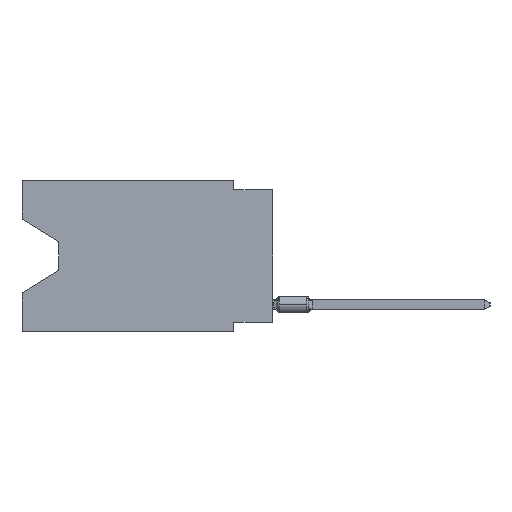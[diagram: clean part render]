
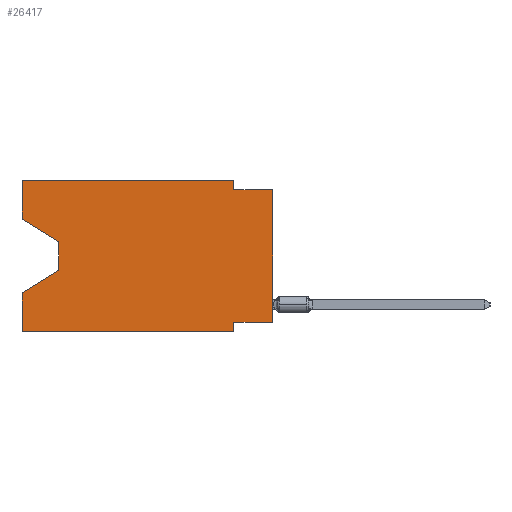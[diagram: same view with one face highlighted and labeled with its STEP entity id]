
A CAD part, left-side view. The second image highlights one B-rep face of the part: STEP entity #26417.
In plain terms, the highlighted planar face has unit normal (-1, 0, 0).
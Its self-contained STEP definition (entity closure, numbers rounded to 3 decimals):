
#156 = EDGE_CURVE ( 'NONE', #57719, #71938, #12240, .T. ) ;
#2306 = LINE ( 'NONE', #27780, #50299 ) ;
#2525 = ORIENTED_EDGE ( 'NONE', *, *, #41939, .F. ) ;
#5189 = DIRECTION ( 'NONE',  ( 0., 0.855, -0.519 ) ) ;
#5828 = ORIENTED_EDGE ( 'NONE', *, *, #59605, .T. ) ;
#7001 = ORIENTED_EDGE ( 'NONE', *, *, #48539, .F. ) ;
#7653 = LINE ( 'NONE', #45884, #35187 ) ;
#9067 = FACE_OUTER_BOUND ( 'NONE', #17213, .T. ) ;
#9467 = VECTOR ( 'NONE', #25848, 1000. ) ;
#11030 = ORIENTED_EDGE ( 'NONE', *, *, #156, .F. ) ;
#12240 = LINE ( 'NONE', #48857, #57373 ) ;
#13187 = AXIS2_PLACEMENT_3D ( 'NONE', #33749, #78529, #22192 ) ;
#14159 = CARTESIAN_POINT ( 'NONE',  ( 0., 2.54, -9.271 ) ) ;
#14435 = ORIENTED_EDGE ( 'NONE', *, *, #80233, .F. ) ;
#14688 = VECTOR ( 'NONE', #21232, 1000. ) ;
#15600 = EDGE_CURVE ( 'NONE', #22724, #71679, #7653, .T. ) ;
#17213 = EDGE_LOOP ( 'NONE', ( #37567, #21564, #76648, #43683, #5828, #53426, #14435, #63205, #7001, #18135, #11030, #2525 ) ) ;
#17422 = CARTESIAN_POINT ( 'NONE',  ( 0., 0., -0.635 ) ) ;
#18135 = ORIENTED_EDGE ( 'NONE', *, *, #28341, .F. ) ;
#18317 = VERTEX_POINT ( 'NONE', #50794 ) ;
#19525 = CARTESIAN_POINT ( 'NONE',  ( 0., 13.97, -5.893 ) ) ;
#21232 = DIRECTION ( 'NONE',  ( 0., -1., 0. ) ) ;
#21564 = ORIENTED_EDGE ( 'NONE', *, *, #15600, .T. ) ;
#22192 = DIRECTION ( 'NONE',  ( 0., 0., -1. ) ) ;
#22479 = VERTEX_POINT ( 'NONE', #40797 ) ;
#22724 = VERTEX_POINT ( 'NONE', #30096 ) ;
#23611 = LINE ( 'NONE', #62969, #29128 ) ;
#25848 = DIRECTION ( 'NONE',  ( 0., 1., 0. ) ) ;
#26417 = ADVANCED_FACE ( 'NONE', ( #9067 ), #34574, .F. ) ;
#26924 = VERTEX_POINT ( 'NONE', #67742 ) ;
#27170 = VECTOR ( 'NONE', #46002, 1000. ) ;
#27328 = EDGE_CURVE ( 'NONE', #54242, #44388, #79955, .T. ) ;
#27780 = CARTESIAN_POINT ( 'NONE',  ( 0., 2.54, 0. ) ) ;
#28341 = EDGE_CURVE ( 'NONE', #71938, #22479, #2306, .T. ) ;
#29128 = VECTOR ( 'NONE', #67624, 1000. ) ;
#29973 = DIRECTION ( 'NONE',  ( 0., 0., 1. ) ) ;
#30096 = CARTESIAN_POINT ( 'NONE',  ( 0., 13.97, -4.013 ) ) ;
#30326 = VECTOR ( 'NONE', #5189, 1000. ) ;
#30375 = LINE ( 'NONE', #55885, #58609 ) ;
#33749 = CARTESIAN_POINT ( 'NONE',  ( 0., 16.383, 0. ) ) ;
#34574 = PLANE ( 'NONE',  #13187 ) ;
#35187 = VECTOR ( 'NONE', #70937, 1000. ) ;
#35700 = CARTESIAN_POINT ( 'NONE',  ( 0., 16.383, 0. ) ) ;
#37567 = ORIENTED_EDGE ( 'NONE', *, *, #71541, .T. ) ;
#40445 = VERTEX_POINT ( 'NONE', #52139 ) ;
#40797 = CARTESIAN_POINT ( 'NONE',  ( 0., 2.54, -0.635 ) ) ;
#41347 = CARTESIAN_POINT ( 'NONE',  ( 0., 2.54, -9.906 ) ) ;
#41939 = EDGE_CURVE ( 'NONE', #18317, #57719, #73947, .T. ) ;
#43683 = ORIENTED_EDGE ( 'NONE', *, *, #71610, .F. ) ;
#44388 = VERTEX_POINT ( 'NONE', #76986 ) ;
#44770 = CARTESIAN_POINT ( 'NONE',  ( 0., 0., -9.271 ) ) ;
#45143 = CARTESIAN_POINT ( 'NONE',  ( 0., 13.97, -5.893 ) ) ;
#45884 = CARTESIAN_POINT ( 'NONE',  ( 0., 13.97, -4.013 ) ) ;
#46002 = DIRECTION ( 'NONE',  ( 0., -1., 0. ) ) ;
#46187 = VERTEX_POINT ( 'NONE', #73726 ) ;
#46312 = DIRECTION ( 'NONE',  ( 0., 0., -1. ) ) ;
#48486 = DIRECTION ( 'NONE',  ( 0., -0.855, -0.519 ) ) ;
#48539 = EDGE_CURVE ( 'NONE', #22479, #46187, #59079, .T. ) ;
#48857 = CARTESIAN_POINT ( 'NONE',  ( 0., 16.383, 0. ) ) ;
#50299 = VECTOR ( 'NONE', #46312, 1000. ) ;
#50565 = LINE ( 'NONE', #44770, #9467 ) ;
#50794 = CARTESIAN_POINT ( 'NONE',  ( 0., 16.383, -2.546 ) ) ;
#50810 = LINE ( 'NONE', #19525, #30326 ) ;
#52139 = CARTESIAN_POINT ( 'NONE',  ( 0., 0., -9.271 ) ) ;
#53426 = ORIENTED_EDGE ( 'NONE', *, *, #27328, .F. ) ;
#54242 = VERTEX_POINT ( 'NONE', #14159 ) ;
#55043 = DIRECTION ( 'NONE',  ( 0., -1., 0. ) ) ;
#55369 = VERTEX_POINT ( 'NONE', #76809 ) ;
#55885 = CARTESIAN_POINT ( 'NONE',  ( 0., 16.383, 0. ) ) ;
#57373 = VECTOR ( 'NONE', #55043, 1000. ) ;
#57719 = VERTEX_POINT ( 'NONE', #35700 ) ;
#58609 = VECTOR ( 'NONE', #75573, 1000. ) ;
#59079 = LINE ( 'NONE', #17422, #14688 ) ;
#59605 = EDGE_CURVE ( 'NONE', #26924, #44388, #71885, .T. ) ;
#60393 = CARTESIAN_POINT ( 'NONE',  ( 0., 16.383, -2.546 ) ) ;
#62969 = CARTESIAN_POINT ( 'NONE',  ( 0., 0., 0. ) ) ;
#63205 = ORIENTED_EDGE ( 'NONE', *, *, #79670, .T. ) ;
#64166 = EDGE_CURVE ( 'NONE', #71679, #55369, #50810, .T. ) ;
#64637 = VECTOR ( 'NONE', #48486, 1000. ) ;
#67624 = DIRECTION ( 'NONE',  ( 0., 0., 1. ) ) ;
#67742 = CARTESIAN_POINT ( 'NONE',  ( 0., 16.383, -9.906 ) ) ;
#69875 = VECTOR ( 'NONE', #71770, 1000. ) ;
#70937 = DIRECTION ( 'NONE',  ( 0., 0., -1. ) ) ;
#71541 = EDGE_CURVE ( 'NONE', #18317, #22724, #79317, .T. ) ;
#71610 = EDGE_CURVE ( 'NONE', #26924, #55369, #30375, .T. ) ;
#71679 = VERTEX_POINT ( 'NONE', #45143 ) ;
#71770 = DIRECTION ( 'NONE',  ( 0., 0., -1. ) ) ;
#71885 = LINE ( 'NONE', #77235, #27170 ) ;
#71938 = VERTEX_POINT ( 'NONE', #73850 ) ;
#73726 = CARTESIAN_POINT ( 'NONE',  ( 0., 0., -0.635 ) ) ;
#73850 = CARTESIAN_POINT ( 'NONE',  ( 0., 2.54, 0. ) ) ;
#73947 = LINE ( 'NONE', #78891, #77682 ) ;
#75573 = DIRECTION ( 'NONE',  ( 0., 0., 1. ) ) ;
#76648 = ORIENTED_EDGE ( 'NONE', *, *, #64166, .T. ) ;
#76809 = CARTESIAN_POINT ( 'NONE',  ( 0., 16.383, -7.36 ) ) ;
#76986 = CARTESIAN_POINT ( 'NONE',  ( 0., 2.54, -9.906 ) ) ;
#77235 = CARTESIAN_POINT ( 'NONE',  ( 0., 16.383, -9.906 ) ) ;
#77682 = VECTOR ( 'NONE', #29973, 1000. ) ;
#78529 = DIRECTION ( 'NONE',  ( 1., 0., 0. ) ) ;
#78891 = CARTESIAN_POINT ( 'NONE',  ( 0., 16.383, 0. ) ) ;
#79317 = LINE ( 'NONE', #60393, #64637 ) ;
#79670 = EDGE_CURVE ( 'NONE', #40445, #46187, #23611, .T. ) ;
#79955 = LINE ( 'NONE', #41347, #69875 ) ;
#80233 = EDGE_CURVE ( 'NONE', #40445, #54242, #50565, .T. ) ;
